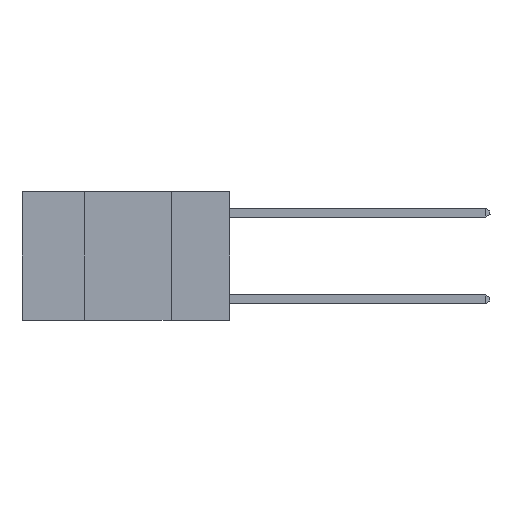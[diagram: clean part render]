
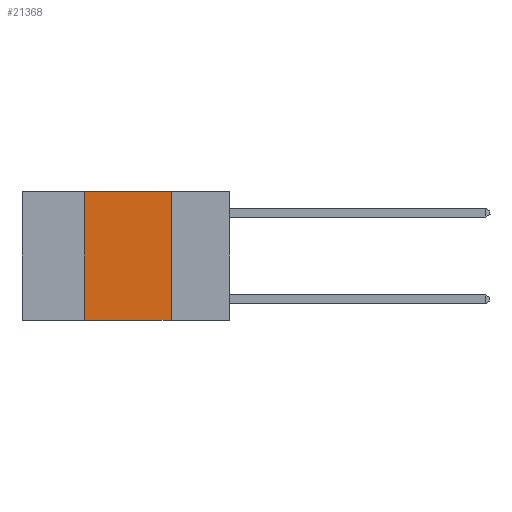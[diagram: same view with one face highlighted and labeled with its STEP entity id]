
A CAD part, left-side view. The second image highlights one B-rep face of the part: STEP entity #21368.
In plain terms, the highlighted planar face has unit normal (-1, 0, 0).
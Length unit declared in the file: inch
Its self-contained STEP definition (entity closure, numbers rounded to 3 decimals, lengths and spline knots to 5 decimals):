
#238 = VERTEX_POINT ( 'NONE', #14436 ) ;
#1478 = DIRECTION ( 'NONE',  ( 1., 0., 0. ) ) ;
#2378 = ORIENTED_EDGE ( 'NONE', *, *, #4106, .F. ) ;
#2437 = DIRECTION ( 'NONE',  ( 0., -1., 0. ) ) ;
#3719 = LINE ( 'NONE', #5479, #5087 ) ;
#4106 = EDGE_CURVE ( 'NONE', #12603, #6597, #20774, .T. ) ;
#4611 = CARTESIAN_POINT ( 'NONE',  ( 0., 0.17, 0. ) ) ;
#4657 = PLANE ( 'NONE',  #18602 ) ;
#5087 = VECTOR ( 'NONE', #19034, 39.37008 ) ;
#5278 = DIRECTION ( 'NONE',  ( 0., 0., -1. ) ) ;
#5479 = CARTESIAN_POINT ( 'NONE',  ( 0., 0.42, 0. ) ) ;
#5499 = EDGE_CURVE ( 'NONE', #238, #12603, #17182, .T. ) ;
#5841 = CARTESIAN_POINT ( 'NONE',  ( 0., 0.6, -0.37 ) ) ;
#6597 = VERTEX_POINT ( 'NONE', #12005 ) ;
#7795 = VECTOR ( 'NONE', #18723, 39.37008 ) ;
#7907 = ORIENTED_EDGE ( 'NONE', *, *, #12494, .T. ) ;
#9088 = VECTOR ( 'NONE', #5278, 39.37008 ) ;
#9852 = VECTOR ( 'NONE', #2437, 39.37008 ) ;
#10972 = CARTESIAN_POINT ( 'NONE',  ( 0., 0.42, -0.37 ) ) ;
#11419 = EDGE_CURVE ( 'NONE', #20880, #238, #3719, .T. ) ;
#12005 = CARTESIAN_POINT ( 'NONE',  ( 0., 0.17, -0.37 ) ) ;
#12494 = EDGE_CURVE ( 'NONE', #20880, #6597, #14519, .T. ) ;
#12603 = VERTEX_POINT ( 'NONE', #4611 ) ;
#14282 = CARTESIAN_POINT ( 'NONE',  ( 0., 0.17, 0. ) ) ;
#14436 = CARTESIAN_POINT ( 'NONE',  ( 0., 0.42, 0. ) ) ;
#14519 = LINE ( 'NONE', #5841, #9852 ) ;
#17182 = LINE ( 'NONE', #20222, #7795 ) ;
#17493 = ORIENTED_EDGE ( 'NONE', *, *, #11419, .F. ) ;
#18218 = CARTESIAN_POINT ( 'NONE',  ( 0., 0.6, 0. ) ) ;
#18330 = FACE_OUTER_BOUND ( 'NONE', #19014, .T. ) ;
#18602 = AXIS2_PLACEMENT_3D ( 'NONE', #18218, #1478, #21577 ) ;
#18723 = DIRECTION ( 'NONE',  ( 0., -1., 0. ) ) ;
#19014 = EDGE_LOOP ( 'NONE', ( #2378, #20238, #17493, #7907 ) ) ;
#19034 = DIRECTION ( 'NONE',  ( 0., 0., 1. ) ) ;
#20222 = CARTESIAN_POINT ( 'NONE',  ( 0., 0.6, 0. ) ) ;
#20238 = ORIENTED_EDGE ( 'NONE', *, *, #5499, .F. ) ;
#20774 = LINE ( 'NONE', #14282, #9088 ) ;
#20880 = VERTEX_POINT ( 'NONE', #10972 ) ;
#21368 = ADVANCED_FACE ( 'NONE', ( #18330 ), #4657, .F. ) ;
#21577 = DIRECTION ( 'NONE',  ( 0., 0., -1. ) ) ;
